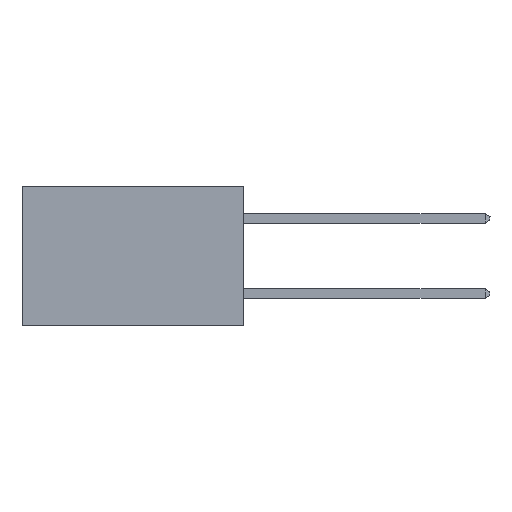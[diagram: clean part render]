
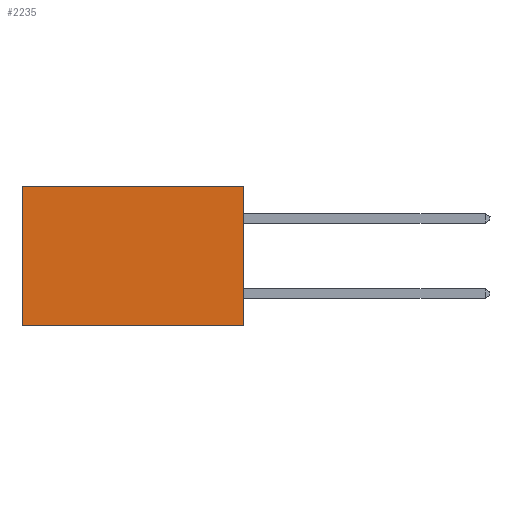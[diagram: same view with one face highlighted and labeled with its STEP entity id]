
A CAD part, left-side view. The second image highlights one B-rep face of the part: STEP entity #2235.
In plain terms, the highlighted planar face has unit normal (-1, 0, 0).
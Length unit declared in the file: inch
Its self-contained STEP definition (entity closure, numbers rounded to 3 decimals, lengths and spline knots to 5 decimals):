
#967 = DIRECTION ( 'NONE',  ( 0., 1., 0. ) ) ;
#1215 = ORIENTED_EDGE ( 'NONE', *, *, #5268, .F. ) ;
#1357 = VERTEX_POINT ( 'NONE', #4153 ) ;
#1534 = CARTESIAN_POINT ( 'NONE',  ( 0.277, 0., 0. ) ) ;
#1561 = DIRECTION ( 'NONE',  ( 0., 1., 0. ) ) ;
#1588 = EDGE_CURVE ( 'NONE', #2157, #1357, #7992, .T. ) ;
#1722 = FACE_OUTER_BOUND ( 'NONE', #6658, .T. ) ;
#1785 = VECTOR ( 'NONE', #967, 39.37008 ) ;
#2157 = VERTEX_POINT ( 'NONE', #7164 ) ;
#2235 = ADVANCED_FACE ( 'NONE', ( #1722 ), #7075, .F. ) ;
#2534 = CARTESIAN_POINT ( 'NONE',  ( 0.277, 0., -0.37 ) ) ;
#2834 = VECTOR ( 'NONE', #1561, 39.37008 ) ;
#2854 = ORIENTED_EDGE ( 'NONE', *, *, #1588, .T. ) ;
#3025 = CARTESIAN_POINT ( 'NONE',  ( 0.277, 0.59, -0.37 ) ) ;
#3099 = ORIENTED_EDGE ( 'NONE', *, *, #5070, .T. ) ;
#3197 = VECTOR ( 'NONE', #6353, 39.37008 ) ;
#3343 = EDGE_CURVE ( 'NONE', #4521, #1357, #5411, .T. ) ;
#3629 = VERTEX_POINT ( 'NONE', #7627 ) ;
#3877 = CARTESIAN_POINT ( 'NONE',  ( 0.277, 0., -0.37 ) ) ;
#4153 = CARTESIAN_POINT ( 'NONE',  ( 0.277, 0.59, -0.37 ) ) ;
#4521 = VERTEX_POINT ( 'NONE', #3877 ) ;
#4606 = ORIENTED_EDGE ( 'NONE', *, *, #3343, .F. ) ;
#5070 = EDGE_CURVE ( 'NONE', #3629, #2157, #8023, .T. ) ;
#5110 = DIRECTION ( 'NONE',  ( 0., 0., -1. ) ) ;
#5268 = EDGE_CURVE ( 'NONE', #3629, #4521, #8295, .T. ) ;
#5411 = LINE ( 'NONE', #2534, #1785 ) ;
#6034 = DIRECTION ( 'NONE',  ( 0., 0., -1. ) ) ;
#6129 = AXIS2_PLACEMENT_3D ( 'NONE', #7727, #6281, #6034 ) ;
#6261 = VECTOR ( 'NONE', #5110, 39.37008 ) ;
#6281 = DIRECTION ( 'NONE',  ( 1., 0., 0. ) ) ;
#6353 = DIRECTION ( 'NONE',  ( 0., 0., -1. ) ) ;
#6364 = CARTESIAN_POINT ( 'NONE',  ( 0.277, 0., -0.37 ) ) ;
#6658 = EDGE_LOOP ( 'NONE', ( #2854, #4606, #1215, #3099 ) ) ;
#7075 = PLANE ( 'NONE',  #6129 ) ;
#7164 = CARTESIAN_POINT ( 'NONE',  ( 0.277, 0.59, 0. ) ) ;
#7627 = CARTESIAN_POINT ( 'NONE',  ( 0.277, 0., 0. ) ) ;
#7727 = CARTESIAN_POINT ( 'NONE',  ( 0.277, 0., -0.37 ) ) ;
#7992 = LINE ( 'NONE', #3025, #6261 ) ;
#8023 = LINE ( 'NONE', #1534, #2834 ) ;
#8295 = LINE ( 'NONE', #6364, #3197 ) ;
